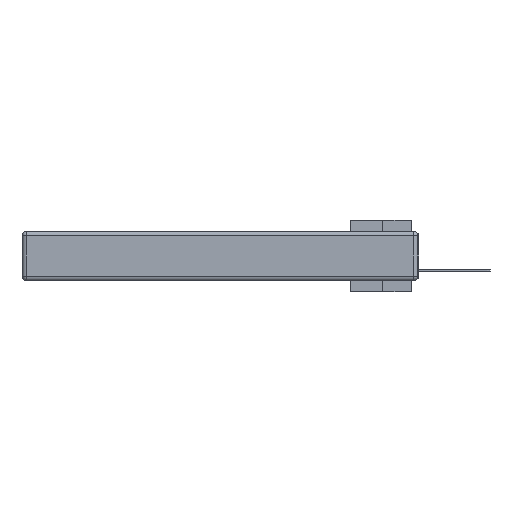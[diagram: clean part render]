
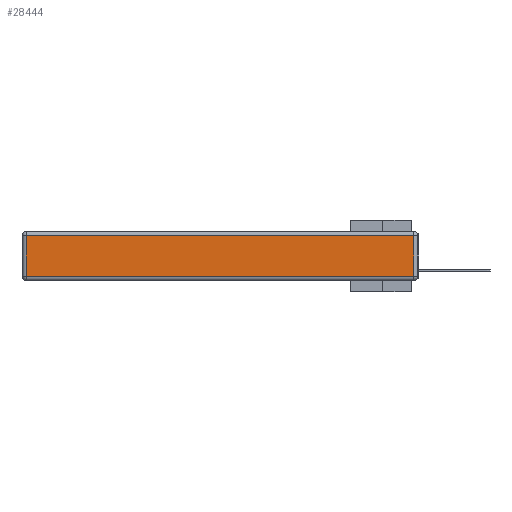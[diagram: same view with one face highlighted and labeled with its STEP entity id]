
A CAD part, left-side view. The second image highlights one B-rep face of the part: STEP entity #28444.
In plain terms, the highlighted planar face has unit normal (-1, 0, 0).
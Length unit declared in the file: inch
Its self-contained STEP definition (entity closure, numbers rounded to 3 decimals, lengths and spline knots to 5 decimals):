
#219 = VECTOR ( 'NONE', #11325, 39.37008 ) ;
#3192 = PLANE ( 'NONE',  #9875 ) ;
#3792 = ORIENTED_EDGE ( 'NONE', *, *, #9417, .T. ) ;
#5279 = EDGE_LOOP ( 'NONE', ( #20740, #15938, #15540, #3792 ) ) ;
#5986 = VERTEX_POINT ( 'NONE', #7820 ) ;
#6307 = VECTOR ( 'NONE', #7419, 39.37008 ) ;
#7419 = DIRECTION ( 'NONE',  ( 0., 0., -1. ) ) ;
#7820 = CARTESIAN_POINT ( 'NONE',  ( 0., 0.03, -0.313 ) ) ;
#9417 = EDGE_CURVE ( 'NONE', #38114, #16766, #16527, .T. ) ;
#9875 = AXIS2_PLACEMENT_3D ( 'NONE', #12285, #12420, #25157 ) ;
#10027 = CARTESIAN_POINT ( 'NONE',  ( 0., 2.72, -0.03 ) ) ;
#10464 = VECTOR ( 'NONE', #13655, 39.37008 ) ;
#11325 = DIRECTION ( 'NONE',  ( 0., -1., 0. ) ) ;
#12285 = CARTESIAN_POINT ( 'NONE',  ( 0., 0., -0.343 ) ) ;
#12420 = DIRECTION ( 'NONE',  ( -1., 0., 0. ) ) ;
#13655 = DIRECTION ( 'NONE',  ( 0., 0., 1. ) ) ;
#14571 = CARTESIAN_POINT ( 'NONE',  ( 0., 0., -0.313 ) ) ;
#15540 = ORIENTED_EDGE ( 'NONE', *, *, #24474, .T. ) ;
#15938 = ORIENTED_EDGE ( 'NONE', *, *, #26671, .T. ) ;
#16527 = LINE ( 'NONE', #19624, #6307 ) ;
#16766 = VERTEX_POINT ( 'NONE', #28851 ) ;
#18698 = LINE ( 'NONE', #14571, #219 ) ;
#19619 = CARTESIAN_POINT ( 'NONE',  ( 0., 0.03, -0.343 ) ) ;
#19624 = CARTESIAN_POINT ( 'NONE',  ( 0., 2.72, -0.343 ) ) ;
#20677 = CARTESIAN_POINT ( 'NONE',  ( 0., 0.03, -0.03 ) ) ;
#20740 = ORIENTED_EDGE ( 'NONE', *, *, #21332, .T. ) ;
#21332 = EDGE_CURVE ( 'NONE', #16766, #5986, #18698, .T. ) ;
#23320 = VERTEX_POINT ( 'NONE', #20677 ) ;
#23623 = LINE ( 'NONE', #19619, #10464 ) ;
#24474 = EDGE_CURVE ( 'NONE', #23320, #38114, #37176, .T. ) ;
#25157 = DIRECTION ( 'NONE',  ( 0., 0., 1. ) ) ;
#26671 = EDGE_CURVE ( 'NONE', #5986, #23320, #23623, .T. ) ;
#27434 = CARTESIAN_POINT ( 'NONE',  ( 0., 2.75, -0.03 ) ) ;
#28444 = ADVANCED_FACE ( 'NONE', ( #38935 ), #3192, .T. ) ;
#28851 = CARTESIAN_POINT ( 'NONE',  ( 0., 2.72, -0.313 ) ) ;
#36217 = VECTOR ( 'NONE', #38867, 39.37008 ) ;
#37176 = LINE ( 'NONE', #27434, #36217 ) ;
#38114 = VERTEX_POINT ( 'NONE', #10027 ) ;
#38867 = DIRECTION ( 'NONE',  ( 0., 1., 0. ) ) ;
#38935 = FACE_OUTER_BOUND ( 'NONE', #5279, .T. ) ;
